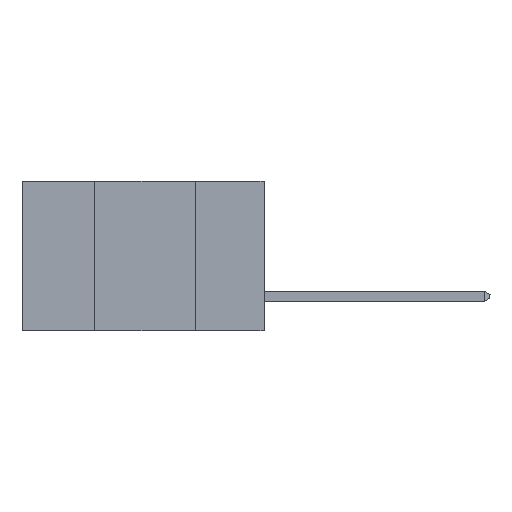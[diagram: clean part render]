
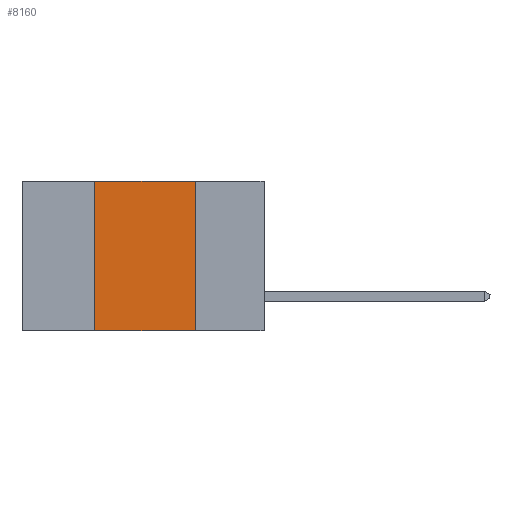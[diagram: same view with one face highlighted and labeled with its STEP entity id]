
A CAD part, left-side view. The second image highlights one B-rep face of the part: STEP entity #8160.
In plain terms, the highlighted planar face has unit normal (-1, 0, 0).
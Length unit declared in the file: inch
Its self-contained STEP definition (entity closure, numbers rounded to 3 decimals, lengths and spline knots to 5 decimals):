
#670 = CARTESIAN_POINT ( 'NONE',  ( 0., 0.6, 0. ) ) ;
#956 = EDGE_LOOP ( 'NONE', ( #4520, #11409, #5901, #12084 ) ) ;
#1462 = DIRECTION ( 'NONE',  ( 0., -1., 0. ) ) ;
#2215 = EDGE_CURVE ( 'NONE', #13659, #6441, #6648, .T. ) ;
#2603 = CARTESIAN_POINT ( 'NONE',  ( 0., 0.6, -0.37 ) ) ;
#3490 = CARTESIAN_POINT ( 'NONE',  ( 0., 0.42, 0. ) ) ;
#3627 = CARTESIAN_POINT ( 'NONE',  ( 0., 0.42, -0.37 ) ) ;
#4010 = PLANE ( 'NONE',  #7066 ) ;
#4504 = DIRECTION ( 'NONE',  ( 0., 0., 1. ) ) ;
#4520 = ORIENTED_EDGE ( 'NONE', *, *, #5388, .F. ) ;
#4858 = VERTEX_POINT ( 'NONE', #7505 ) ;
#5199 = DIRECTION ( 'NONE',  ( 0., 0., -1. ) ) ;
#5388 = EDGE_CURVE ( 'NONE', #6441, #4858, #9084, .T. ) ;
#5771 = VERTEX_POINT ( 'NONE', #3627 ) ;
#5901 = ORIENTED_EDGE ( 'NONE', *, *, #9332, .F. ) ;
#6441 = VERTEX_POINT ( 'NONE', #7978 ) ;
#6648 = LINE ( 'NONE', #7763, #11466 ) ;
#6757 = VECTOR ( 'NONE', #1462, 39.37008 ) ;
#7066 = AXIS2_PLACEMENT_3D ( 'NONE', #670, #12366, #10976 ) ;
#7505 = CARTESIAN_POINT ( 'NONE',  ( 0., 0.17, -0.37 ) ) ;
#7763 = CARTESIAN_POINT ( 'NONE',  ( 0., 0.6, 0. ) ) ;
#7978 = CARTESIAN_POINT ( 'NONE',  ( 0., 0.17, 0. ) ) ;
#8160 = ADVANCED_FACE ( 'NONE', ( #14219 ), #4010, .F. ) ;
#9084 = LINE ( 'NONE', #12379, #10149 ) ;
#9332 = EDGE_CURVE ( 'NONE', #5771, #13659, #12579, .T. ) ;
#10149 = VECTOR ( 'NONE', #5199, 39.37008 ) ;
#10976 = DIRECTION ( 'NONE',  ( 0., 0., -1. ) ) ;
#11409 = ORIENTED_EDGE ( 'NONE', *, *, #2215, .F. ) ;
#11466 = VECTOR ( 'NONE', #13461, 39.37008 ) ;
#12084 = ORIENTED_EDGE ( 'NONE', *, *, #13128, .T. ) ;
#12366 = DIRECTION ( 'NONE',  ( 1., 0., 0. ) ) ;
#12379 = CARTESIAN_POINT ( 'NONE',  ( 0., 0.17, 0. ) ) ;
#12392 = VECTOR ( 'NONE', #4504, 39.37008 ) ;
#12579 = LINE ( 'NONE', #13656, #12392 ) ;
#12996 = LINE ( 'NONE', #2603, #6757 ) ;
#13128 = EDGE_CURVE ( 'NONE', #5771, #4858, #12996, .T. ) ;
#13461 = DIRECTION ( 'NONE',  ( 0., -1., 0. ) ) ;
#13656 = CARTESIAN_POINT ( 'NONE',  ( 0., 0.42, 0. ) ) ;
#13659 = VERTEX_POINT ( 'NONE', #3490 ) ;
#14219 = FACE_OUTER_BOUND ( 'NONE', #956, .T. ) ;
